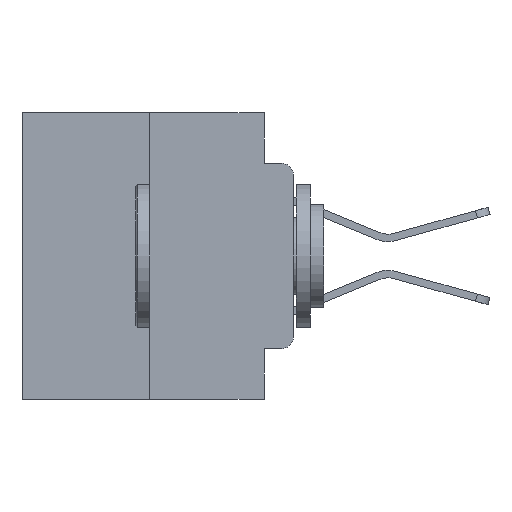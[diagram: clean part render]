
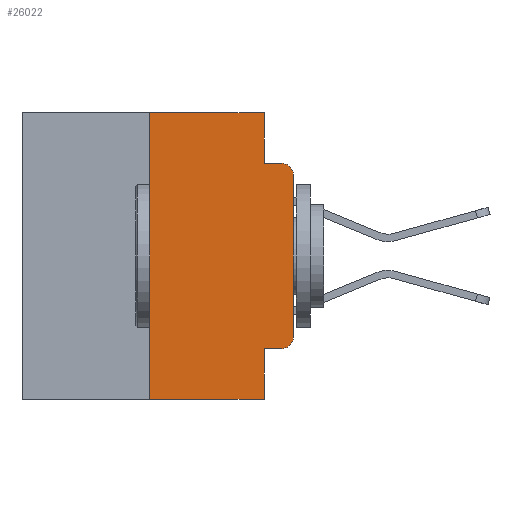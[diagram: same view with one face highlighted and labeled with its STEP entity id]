
A CAD part, left-side view. The second image highlights one B-rep face of the part: STEP entity #26022.
In plain terms, the highlighted planar face has unit normal (-1, 0, 0).
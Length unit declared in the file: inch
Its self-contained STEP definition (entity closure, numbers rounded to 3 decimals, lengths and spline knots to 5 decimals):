
#262 = VERTEX_POINT ( 'NONE', #6310 ) ;
#337 = CARTESIAN_POINT ( 'NONE',  ( 0., 0.25, -0.5 ) ) ;
#973 = DIRECTION ( 'NONE',  ( 0., 0., -1. ) ) ;
#1362 = AXIS2_PLACEMENT_3D ( 'NONE', #5356, #11969, #26922 ) ;
#1586 = ORIENTED_EDGE ( 'NONE', *, *, #12741, .F. ) ;
#1696 = DIRECTION ( 'NONE',  ( 0., -1., 0. ) ) ;
#1810 = EDGE_CURVE ( 'NONE', #10223, #14523, #6189, .T. ) ;
#1833 = CARTESIAN_POINT ( 'NONE',  ( 0., 0.02, -0.3915 ) ) ;
#2139 = CARTESIAN_POINT ( 'NONE',  ( 0., 0.25, 0. ) ) ;
#4018 = DIRECTION ( 'NONE',  ( 0., 0., 1. ) ) ;
#4108 = DIRECTION ( 'NONE',  ( 0., 0., -1. ) ) ;
#4109 = CARTESIAN_POINT ( 'NONE',  ( 0., 0.051, 0. ) ) ;
#4650 = CARTESIAN_POINT ( 'NONE',  ( 0., 0.02, -0.4115 ) ) ;
#5356 = CARTESIAN_POINT ( 'NONE',  ( 0., 0.473, 0. ) ) ;
#6147 = AXIS2_PLACEMENT_3D ( 'NONE', #27656, #14900, #973 ) ;
#6159 = ORIENTED_EDGE ( 'NONE', *, *, #15672, .T. ) ;
#6189 = LINE ( 'NONE', #7579, #22776 ) ;
#6220 = CARTESIAN_POINT ( 'NONE',  ( 0., 0.051, -0.0885 ) ) ;
#6244 = LINE ( 'NONE', #4109, #22825 ) ;
#6310 = CARTESIAN_POINT ( 'NONE',  ( 0., 0.051, -0.0885 ) ) ;
#6339 = CARTESIAN_POINT ( 'NONE',  ( 0., 0.473, -0.5 ) ) ;
#6590 = LINE ( 'NONE', #22518, #16765 ) ;
#6898 = EDGE_CURVE ( 'NONE', #20958, #262, #19853, .T. ) ;
#6913 = VERTEX_POINT ( 'NONE', #2139 ) ;
#7579 = CARTESIAN_POINT ( 'NONE',  ( 0., 0.051, -0.4115 ) ) ;
#7582 = ORIENTED_EDGE ( 'NONE', *, *, #1810, .T. ) ;
#7970 = VERTEX_POINT ( 'NONE', #25153 ) ;
#8413 = FACE_OUTER_BOUND ( 'NONE', #23630, .T. ) ;
#8846 = CIRCLE ( 'NONE', #6147, 0.02 ) ;
#9293 = ORIENTED_EDGE ( 'NONE', *, *, #20364, .T. ) ;
#9331 = EDGE_CURVE ( 'NONE', #262, #12786, #15614, .T. ) ;
#9699 = VERTEX_POINT ( 'NONE', #25061 ) ;
#9855 = EDGE_CURVE ( 'NONE', #19446, #6913, #13572, .T. ) ;
#10223 = VERTEX_POINT ( 'NONE', #26794 ) ;
#10548 = EDGE_CURVE ( 'NONE', #14523, #9699, #23901, .T. ) ;
#10972 = CARTESIAN_POINT ( 'NONE',  ( 0., 0.051, 0. ) ) ;
#11723 = CARTESIAN_POINT ( 'NONE',  ( 0., 0.051, 0. ) ) ;
#11969 = DIRECTION ( 'NONE',  ( 1., 0., 0. ) ) ;
#12741 = EDGE_CURVE ( 'NONE', #10223, #7970, #6244, .T. ) ;
#12786 = VERTEX_POINT ( 'NONE', #21691 ) ;
#13572 = LINE ( 'NONE', #14962, #18597 ) ;
#14147 = VECTOR ( 'NONE', #17449, 39.37008 ) ;
#14523 = VERTEX_POINT ( 'NONE', #4650 ) ;
#14900 = DIRECTION ( 'NONE',  ( -1., 0., 0. ) ) ;
#14931 = CARTESIAN_POINT ( 'NONE',  ( 0., 0., 0. ) ) ;
#14962 = CARTESIAN_POINT ( 'NONE',  ( 0., 0.25, 0. ) ) ;
#15006 = ORIENTED_EDGE ( 'NONE', *, *, #9331, .F. ) ;
#15261 = LINE ( 'NONE', #6339, #20318 ) ;
#15614 = LINE ( 'NONE', #6220, #20669 ) ;
#15672 = EDGE_CURVE ( 'NONE', #19446, #7970, #15261, .T. ) ;
#16043 = DIRECTION ( 'NONE',  ( 0., -1., 0. ) ) ;
#16365 = ORIENTED_EDGE ( 'NONE', *, *, #6898, .F. ) ;
#16765 = VECTOR ( 'NONE', #16043, 39.37008 ) ;
#17105 = DIRECTION ( 'NONE',  ( 0., 0., 1. ) ) ;
#17167 = DIRECTION ( 'NONE',  ( -1., 0., 0. ) ) ;
#17449 = DIRECTION ( 'NONE',  ( 0., 0., -1. ) ) ;
#18424 = CARTESIAN_POINT ( 'NONE',  ( 0., 0., -0.1085 ) ) ;
#18597 = VECTOR ( 'NONE', #17105, 39.37008 ) ;
#19446 = VERTEX_POINT ( 'NONE', #337 ) ;
#19725 = ORIENTED_EDGE ( 'NONE', *, *, #10548, .T. ) ;
#19784 = VECTOR ( 'NONE', #4018, 39.37008 ) ;
#19853 = LINE ( 'NONE', #10972, #14147 ) ;
#20318 = VECTOR ( 'NONE', #23616, 39.37008 ) ;
#20364 = EDGE_CURVE ( 'NONE', #24798, #12786, #8846, .T. ) ;
#20669 = VECTOR ( 'NONE', #1696, 39.37008 ) ;
#20958 = VERTEX_POINT ( 'NONE', #11723 ) ;
#21691 = CARTESIAN_POINT ( 'NONE',  ( 0., 0.02, -0.0885 ) ) ;
#22077 = ORIENTED_EDGE ( 'NONE', *, *, #27264, .F. ) ;
#22518 = CARTESIAN_POINT ( 'NONE',  ( 0., 0.473, 0. ) ) ;
#22676 = PLANE ( 'NONE',  #1362 ) ;
#22776 = VECTOR ( 'NONE', #27295, 39.37008 ) ;
#22825 = VECTOR ( 'NONE', #27942, 39.37008 ) ;
#23225 = EDGE_CURVE ( 'NONE', #9699, #24798, #27417, .T. ) ;
#23616 = DIRECTION ( 'NONE',  ( 0., -1., 0. ) ) ;
#23630 = EDGE_LOOP ( 'NONE', ( #25046, #9293, #15006, #16365, #22077, #27665, #6159, #1586, #7582, #19725 ) ) ;
#23901 = CIRCLE ( 'NONE', #28105, 0.02 ) ;
#24798 = VERTEX_POINT ( 'NONE', #18424 ) ;
#25046 = ORIENTED_EDGE ( 'NONE', *, *, #23225, .T. ) ;
#25061 = CARTESIAN_POINT ( 'NONE',  ( 0., 0., -0.3915 ) ) ;
#25153 = CARTESIAN_POINT ( 'NONE',  ( 0., 0.051, -0.5 ) ) ;
#26022 = ADVANCED_FACE ( 'NONE', ( #8413 ), #22676, .F. ) ;
#26794 = CARTESIAN_POINT ( 'NONE',  ( 0., 0.051, -0.4115 ) ) ;
#26922 = DIRECTION ( 'NONE',  ( 0., 0., -1. ) ) ;
#27264 = EDGE_CURVE ( 'NONE', #6913, #20958, #6590, .T. ) ;
#27295 = DIRECTION ( 'NONE',  ( 0., -1., 0. ) ) ;
#27417 = LINE ( 'NONE', #14931, #19784 ) ;
#27656 = CARTESIAN_POINT ( 'NONE',  ( 0., 0.02, -0.1085 ) ) ;
#27665 = ORIENTED_EDGE ( 'NONE', *, *, #9855, .F. ) ;
#27942 = DIRECTION ( 'NONE',  ( 0., 0., -1. ) ) ;
#28105 = AXIS2_PLACEMENT_3D ( 'NONE', #1833, #17167, #4108 ) ;
